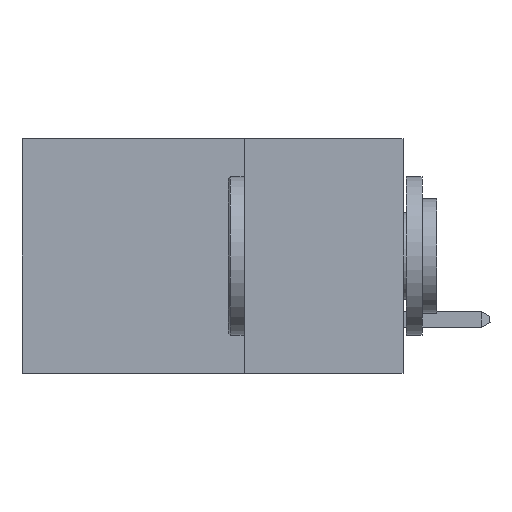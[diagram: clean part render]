
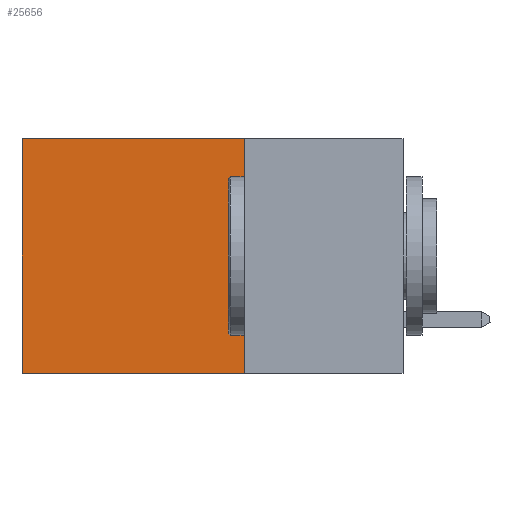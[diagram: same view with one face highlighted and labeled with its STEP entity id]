
A CAD part, left-side view. The second image highlights one B-rep face of the part: STEP entity #25656.
In plain terms, the highlighted planar face has unit normal (-1, 0, 0).
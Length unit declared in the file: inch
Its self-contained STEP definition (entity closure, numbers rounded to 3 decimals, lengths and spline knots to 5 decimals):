
#1102 = CARTESIAN_POINT ( 'NONE',  ( 0.2875, 0.6, 0. ) ) ;
#2955 = LINE ( 'NONE', #15053, #27148 ) ;
#3046 = AXIS2_PLACEMENT_3D ( 'NONE', #35967, #39298, #21803 ) ;
#3391 = CARTESIAN_POINT ( 'NONE',  ( 0.2875, 0.6, 0. ) ) ;
#5874 = ORIENTED_EDGE ( 'NONE', *, *, #19307, .T. ) ;
#6105 = DIRECTION ( 'NONE',  ( 0., 1., 0. ) ) ;
#7373 = LINE ( 'NONE', #30300, #29461 ) ;
#8346 = VERTEX_POINT ( 'NONE', #22517 ) ;
#9710 = VERTEX_POINT ( 'NONE', #26363 ) ;
#10898 = LINE ( 'NONE', #18089, #34072 ) ;
#11668 = CARTESIAN_POINT ( 'NONE',  ( 0.2875, 0.6, -0.37 ) ) ;
#12314 = EDGE_CURVE ( 'NONE', #9710, #26374, #10898, .T. ) ;
#14105 = ORIENTED_EDGE ( 'NONE', *, *, #33289, .T. ) ;
#15053 = CARTESIAN_POINT ( 'NONE',  ( 0.2875, 0.25, 0. ) ) ;
#15197 = PLANE ( 'NONE',  #3046 ) ;
#18089 = CARTESIAN_POINT ( 'NONE',  ( 0.2875, 0.25, -0.37 ) ) ;
#19307 = EDGE_CURVE ( 'NONE', #8346, #39375, #7373, .T. ) ;
#21803 = DIRECTION ( 'NONE',  ( 0., 0., -1. ) ) ;
#22517 = CARTESIAN_POINT ( 'NONE',  ( 0.2875, 0.25, 0. ) ) ;
#25130 = ORIENTED_EDGE ( 'NONE', *, *, #12314, .F. ) ;
#25656 = ADVANCED_FACE ( 'NONE', ( #44365 ), #15197, .F. ) ;
#26211 = EDGE_LOOP ( 'NONE', ( #14105, #25130, #37465, #5874 ) ) ;
#26363 = CARTESIAN_POINT ( 'NONE',  ( 0.2875, 0.25, -0.37 ) ) ;
#26374 = VERTEX_POINT ( 'NONE', #11668 ) ;
#27148 = VECTOR ( 'NONE', #31913, 39.37008 ) ;
#27620 = VECTOR ( 'NONE', #30869, 39.37008 ) ;
#29461 = VECTOR ( 'NONE', #6105, 39.37008 ) ;
#30300 = CARTESIAN_POINT ( 'NONE',  ( 0.2875, 0.25, 0. ) ) ;
#30869 = DIRECTION ( 'NONE',  ( 0., 0., -1. ) ) ;
#31913 = DIRECTION ( 'NONE',  ( 0., 0., -1. ) ) ;
#32546 = DIRECTION ( 'NONE',  ( 0., 1., 0. ) ) ;
#33289 = EDGE_CURVE ( 'NONE', #39375, #26374, #43828, .T. ) ;
#34072 = VECTOR ( 'NONE', #32546, 39.37008 ) ;
#35967 = CARTESIAN_POINT ( 'NONE',  ( 0.2875, 0.25, 0. ) ) ;
#37465 = ORIENTED_EDGE ( 'NONE', *, *, #41491, .F. ) ;
#39298 = DIRECTION ( 'NONE',  ( 1., 0., 0. ) ) ;
#39375 = VERTEX_POINT ( 'NONE', #3391 ) ;
#41491 = EDGE_CURVE ( 'NONE', #8346, #9710, #2955, .T. ) ;
#43828 = LINE ( 'NONE', #1102, #27620 ) ;
#44365 = FACE_OUTER_BOUND ( 'NONE', #26211, .T. ) ;
